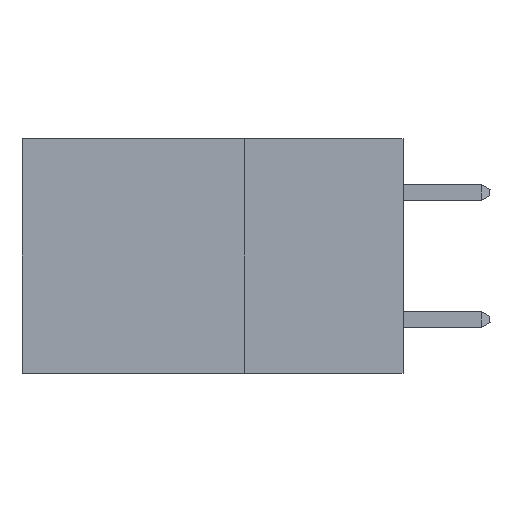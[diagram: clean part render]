
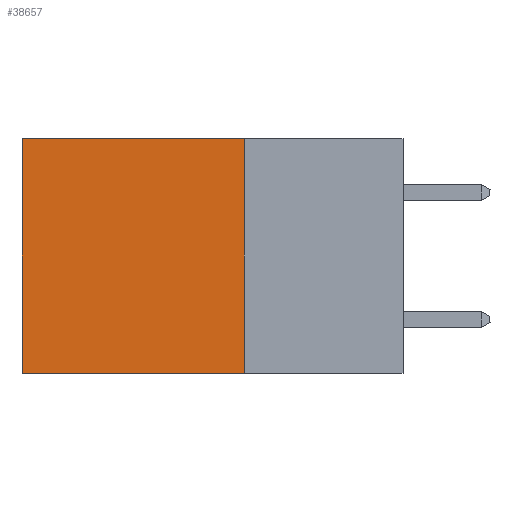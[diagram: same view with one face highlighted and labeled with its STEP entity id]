
A CAD part, left-side view. The second image highlights one B-rep face of the part: STEP entity #38657.
In plain terms, the highlighted planar face has unit normal (-1, 0, 0).
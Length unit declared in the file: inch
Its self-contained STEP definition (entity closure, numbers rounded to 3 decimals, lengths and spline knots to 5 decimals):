
#263 = VECTOR ( 'NONE', #25639, 39.37008 ) ;
#853 = LINE ( 'NONE', #15714, #18176 ) ;
#3488 = DIRECTION ( 'NONE',  ( 0., 0., -1. ) ) ;
#4214 = CARTESIAN_POINT ( 'NONE',  ( 0.2875, 0.6, -0.37 ) ) ;
#4481 = CARTESIAN_POINT ( 'NONE',  ( 0.2875, 0.25, 0. ) ) ;
#4831 = VECTOR ( 'NONE', #12692, 39.37008 ) ;
#5075 = DIRECTION ( 'NONE',  ( 1., 0., 0. ) ) ;
#6750 = CARTESIAN_POINT ( 'NONE',  ( 0.2875, 0.25, 0. ) ) ;
#7379 = ORIENTED_EDGE ( 'NONE', *, *, #21916, .F. ) ;
#8073 = DIRECTION ( 'NONE',  ( 0., 0., -1. ) ) ;
#10205 = ORIENTED_EDGE ( 'NONE', *, *, #13907, .T. ) ;
#11082 = EDGE_LOOP ( 'NONE', ( #10205, #7379, #24161, #35488 ) ) ;
#11410 = EDGE_CURVE ( 'NONE', #17590, #37313, #12359, .T. ) ;
#12359 = LINE ( 'NONE', #6750, #4831 ) ;
#12401 = DIRECTION ( 'NONE',  ( 0., 0., -1. ) ) ;
#12434 = LINE ( 'NONE', #22907, #263 ) ;
#12692 = DIRECTION ( 'NONE',  ( 0., 1., 0. ) ) ;
#13907 = EDGE_CURVE ( 'NONE', #37313, #19210, #35024, .T. ) ;
#13953 = FACE_OUTER_BOUND ( 'NONE', #11082, .T. ) ;
#15714 = CARTESIAN_POINT ( 'NONE',  ( 0.2875, 0.25, 0. ) ) ;
#17590 = VERTEX_POINT ( 'NONE', #4481 ) ;
#18176 = VECTOR ( 'NONE', #3488, 39.37008 ) ;
#19210 = VERTEX_POINT ( 'NONE', #4214 ) ;
#20026 = PLANE ( 'NONE',  #35129 ) ;
#20310 = EDGE_CURVE ( 'NONE', #17590, #38131, #853, .T. ) ;
#21703 = CARTESIAN_POINT ( 'NONE',  ( 0.2875, 0.6, 0. ) ) ;
#21916 = EDGE_CURVE ( 'NONE', #38131, #19210, #12434, .T. ) ;
#22907 = CARTESIAN_POINT ( 'NONE',  ( 0.2875, 0.25, -0.37 ) ) ;
#24161 = ORIENTED_EDGE ( 'NONE', *, *, #20310, .F. ) ;
#25436 = CARTESIAN_POINT ( 'NONE',  ( 0.2875, 0.6, 0. ) ) ;
#25639 = DIRECTION ( 'NONE',  ( 0., 1., 0. ) ) ;
#29466 = VECTOR ( 'NONE', #12401, 39.37008 ) ;
#32966 = CARTESIAN_POINT ( 'NONE',  ( 0.2875, 0.25, -0.37 ) ) ;
#35024 = LINE ( 'NONE', #21703, #29466 ) ;
#35129 = AXIS2_PLACEMENT_3D ( 'NONE', #37776, #5075, #8073 ) ;
#35488 = ORIENTED_EDGE ( 'NONE', *, *, #11410, .T. ) ;
#37313 = VERTEX_POINT ( 'NONE', #25436 ) ;
#37776 = CARTESIAN_POINT ( 'NONE',  ( 0.2875, 0.25, 0. ) ) ;
#38131 = VERTEX_POINT ( 'NONE', #32966 ) ;
#38657 = ADVANCED_FACE ( 'NONE', ( #13953 ), #20026, .F. ) ;
